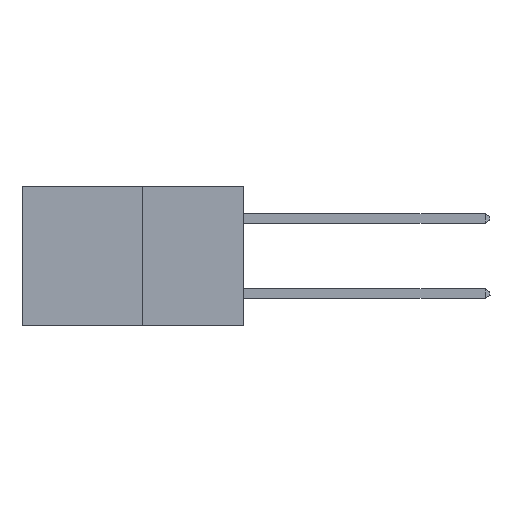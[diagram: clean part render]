
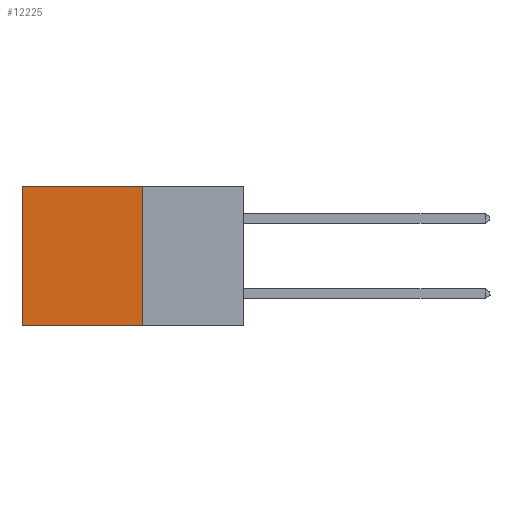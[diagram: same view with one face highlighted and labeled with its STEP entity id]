
A CAD part, left-side view. The second image highlights one B-rep face of the part: STEP entity #12225.
In plain terms, the highlighted planar face has unit normal (-1, 0, 0).
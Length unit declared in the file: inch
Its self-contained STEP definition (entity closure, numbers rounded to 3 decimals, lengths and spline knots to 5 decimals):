
#253 = CARTESIAN_POINT ( 'NONE',  ( 0.277, 0.27, -0.37 ) ) ;
#567 = AXIS2_PLACEMENT_3D ( 'NONE', #4537, #6814, #22592 ) ;
#766 = EDGE_CURVE ( 'NONE', #20216, #2561, #24486, .T. ) ;
#2227 = ORIENTED_EDGE ( 'NONE', *, *, #17950, .F. ) ;
#2561 = VERTEX_POINT ( 'NONE', #20721 ) ;
#2664 = ORIENTED_EDGE ( 'NONE', *, *, #766, .T. ) ;
#4537 = CARTESIAN_POINT ( 'NONE',  ( 0.277, 0.27, -0.37 ) ) ;
#5520 = VERTEX_POINT ( 'NONE', #26756 ) ;
#6814 = DIRECTION ( 'NONE',  ( 1., 0., 0. ) ) ;
#6878 = EDGE_LOOP ( 'NONE', ( #26872, #20062, #2227, #2664 ) ) ;
#7035 = DIRECTION ( 'NONE',  ( 0., 1., 0. ) ) ;
#8648 = FACE_OUTER_BOUND ( 'NONE', #6878, .T. ) ;
#10130 = CARTESIAN_POINT ( 'NONE',  ( 0.277, 0.27, 0. ) ) ;
#10290 = EDGE_CURVE ( 'NONE', #5520, #12840, #13000, .T. ) ;
#11590 = VECTOR ( 'NONE', #7035, 39.37008 ) ;
#12225 = ADVANCED_FACE ( 'NONE', ( #8648 ), #18066, .F. ) ;
#12495 = VECTOR ( 'NONE', #26379, 39.37008 ) ;
#12840 = VERTEX_POINT ( 'NONE', #13199 ) ;
#13000 = LINE ( 'NONE', #253, #11590 ) ;
#13199 = CARTESIAN_POINT ( 'NONE',  ( 0.277, 0.59, -0.37 ) ) ;
#16072 = CARTESIAN_POINT ( 'NONE',  ( 0.277, 0.27, -0.37 ) ) ;
#17539 = VECTOR ( 'NONE', #25016, 39.37008 ) ;
#17950 = EDGE_CURVE ( 'NONE', #20216, #5520, #23556, .T. ) ;
#18066 = PLANE ( 'NONE',  #567 ) ;
#19210 = EDGE_CURVE ( 'NONE', #2561, #12840, #25567, .T. ) ;
#19605 = VECTOR ( 'NONE', #27200, 39.37008 ) ;
#20062 = ORIENTED_EDGE ( 'NONE', *, *, #10290, .F. ) ;
#20185 = CARTESIAN_POINT ( 'NONE',  ( 0.277, 0.59, -0.37 ) ) ;
#20216 = VERTEX_POINT ( 'NONE', #10130 ) ;
#20721 = CARTESIAN_POINT ( 'NONE',  ( 0.277, 0.59, 0. ) ) ;
#22592 = DIRECTION ( 'NONE',  ( 0., 0., -1. ) ) ;
#23556 = LINE ( 'NONE', #16072, #17539 ) ;
#24486 = LINE ( 'NONE', #26825, #12495 ) ;
#25016 = DIRECTION ( 'NONE',  ( 0., 0., -1. ) ) ;
#25567 = LINE ( 'NONE', #20185, #19605 ) ;
#26379 = DIRECTION ( 'NONE',  ( 0., 1., 0. ) ) ;
#26756 = CARTESIAN_POINT ( 'NONE',  ( 0.277, 0.27, -0.37 ) ) ;
#26825 = CARTESIAN_POINT ( 'NONE',  ( 0.277, 0.27, 0. ) ) ;
#26872 = ORIENTED_EDGE ( 'NONE', *, *, #19210, .T. ) ;
#27200 = DIRECTION ( 'NONE',  ( 0., 0., -1. ) ) ;
